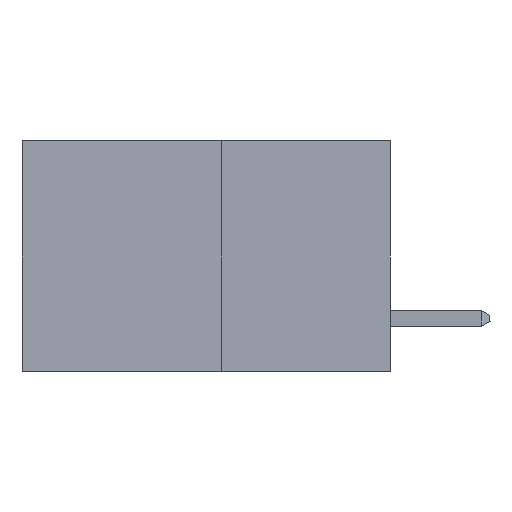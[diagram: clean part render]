
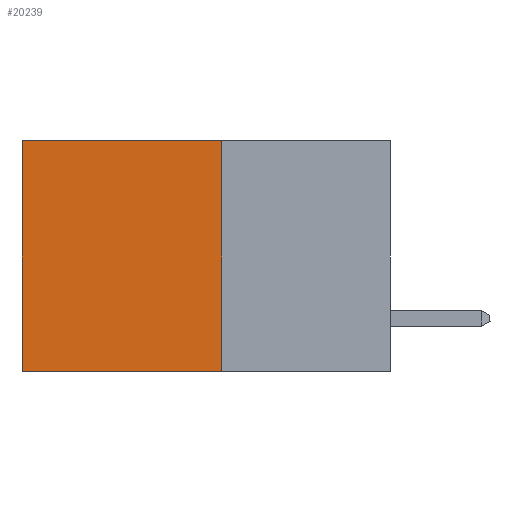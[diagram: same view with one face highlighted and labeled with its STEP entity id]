
A CAD part, left-side view. The second image highlights one B-rep face of the part: STEP entity #20239.
In plain terms, the highlighted planar face has unit normal (-1, 0, 0).
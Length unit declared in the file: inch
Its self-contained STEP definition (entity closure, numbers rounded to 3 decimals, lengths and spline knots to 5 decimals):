
#68 = LINE ( 'NONE', #18143, #3914 ) ;
#276 = CARTESIAN_POINT ( 'NONE',  ( 0.277, 0.27, -0.37 ) ) ;
#948 = FACE_OUTER_BOUND ( 'NONE', #1643, .T. ) ;
#1062 = VECTOR ( 'NONE', #1779, 39.37008 ) ;
#1590 = ORIENTED_EDGE ( 'NONE', *, *, #17864, .F. ) ;
#1643 = EDGE_LOOP ( 'NONE', ( #19705, #1590, #7347, #11754 ) ) ;
#1687 = CARTESIAN_POINT ( 'NONE',  ( 0.277, 0.27, 0. ) ) ;
#1779 = DIRECTION ( 'NONE',  ( 0., 0., -1. ) ) ;
#2199 = CARTESIAN_POINT ( 'NONE',  ( 0.277, 0.27, -0.37 ) ) ;
#2257 = VECTOR ( 'NONE', #6094, 39.37008 ) ;
#3687 = CARTESIAN_POINT ( 'NONE',  ( 0.277, 0.59, 0. ) ) ;
#3788 = LINE ( 'NONE', #17336, #2257 ) ;
#3914 = VECTOR ( 'NONE', #18130, 39.37008 ) ;
#5062 = VERTEX_POINT ( 'NONE', #7822 ) ;
#5175 = VERTEX_POINT ( 'NONE', #276 ) ;
#6094 = DIRECTION ( 'NONE',  ( 0., 1., 0. ) ) ;
#6376 = VERTEX_POINT ( 'NONE', #3687 ) ;
#6403 = LINE ( 'NONE', #13175, #1062 ) ;
#6771 = VECTOR ( 'NONE', #15095, 39.37008 ) ;
#6854 = PLANE ( 'NONE',  #17262 ) ;
#7347 = ORIENTED_EDGE ( 'NONE', *, *, #9201, .F. ) ;
#7822 = CARTESIAN_POINT ( 'NONE',  ( 0.277, 0.59, -0.37 ) ) ;
#9201 = EDGE_CURVE ( 'NONE', #20124, #5175, #68, .T. ) ;
#10190 = DIRECTION ( 'NONE',  ( 0., 0., -1. ) ) ;
#11754 = ORIENTED_EDGE ( 'NONE', *, *, #19941, .T. ) ;
#13175 = CARTESIAN_POINT ( 'NONE',  ( 0.277, 0.59, -0.37 ) ) ;
#14376 = EDGE_CURVE ( 'NONE', #6376, #5062, #6403, .T. ) ;
#15095 = DIRECTION ( 'NONE',  ( 0., 1., 0. ) ) ;
#15898 = LINE ( 'NONE', #2199, #6771 ) ;
#17262 = AXIS2_PLACEMENT_3D ( 'NONE', #18064, #19644, #10190 ) ;
#17336 = CARTESIAN_POINT ( 'NONE',  ( 0.277, 0.27, 0. ) ) ;
#17864 = EDGE_CURVE ( 'NONE', #5175, #5062, #15898, .T. ) ;
#18064 = CARTESIAN_POINT ( 'NONE',  ( 0.277, 0.27, -0.37 ) ) ;
#18130 = DIRECTION ( 'NONE',  ( 0., 0., -1. ) ) ;
#18143 = CARTESIAN_POINT ( 'NONE',  ( 0.277, 0.27, -0.37 ) ) ;
#19644 = DIRECTION ( 'NONE',  ( 1., 0., 0. ) ) ;
#19705 = ORIENTED_EDGE ( 'NONE', *, *, #14376, .T. ) ;
#19941 = EDGE_CURVE ( 'NONE', #20124, #6376, #3788, .T. ) ;
#20124 = VERTEX_POINT ( 'NONE', #1687 ) ;
#20239 = ADVANCED_FACE ( 'NONE', ( #948 ), #6854, .F. ) ;
